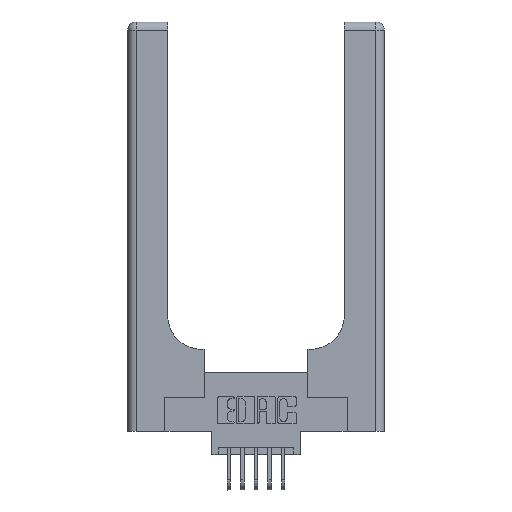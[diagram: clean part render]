
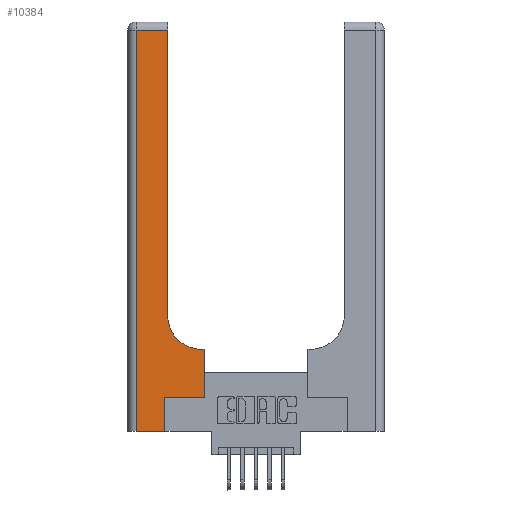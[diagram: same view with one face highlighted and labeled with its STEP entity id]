
A CAD part, top view. The second image highlights one B-rep face of the part: STEP entity #10384.
In plain terms, the highlighted planar face has unit normal (0, 0, 1).
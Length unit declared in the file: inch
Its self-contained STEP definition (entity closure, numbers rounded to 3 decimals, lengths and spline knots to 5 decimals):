
#715 = CARTESIAN_POINT ( 'NONE',  ( 0., 3., 0.37 ) ) ;
#1018 = CARTESIAN_POINT ( 'NONE',  ( 0., 2.94, 0.37 ) ) ;
#1061 = VERTEX_POINT ( 'NONE', #5881 ) ;
#1161 = EDGE_CURVE ( 'NONE', #7354, #1061, #1503, .T. ) ;
#1454 = VERTEX_POINT ( 'NONE', #11573 ) ;
#1472 = VECTOR ( 'NONE', #3896, 39.37008 ) ;
#1502 = CARTESIAN_POINT ( 'NONE',  ( 0.06, 3., 0.37 ) ) ;
#1503 = LINE ( 'NONE', #4188, #1472 ) ;
#1912 = CARTESIAN_POINT ( 'NONE',  ( 0.06, 2.94, 0.37 ) ) ;
#1998 = CARTESIAN_POINT ( 'NONE',  ( 0.269, 0., 0.37 ) ) ;
#2055 = EDGE_CURVE ( 'NONE', #10056, #12913, #4078, .T. ) ;
#2505 = LINE ( 'NONE', #11659, #2764 ) ;
#2760 = CARTESIAN_POINT ( 'NONE',  ( 0.269, 0., 0.37 ) ) ;
#2764 = VECTOR ( 'NONE', #5152, 39.37008 ) ;
#3161 = CARTESIAN_POINT ( 'NONE',  ( 0.5415, 0.85, 0.37 ) ) ;
#3409 = ORIENTED_EDGE ( 'NONE', *, *, #1161, .T. ) ;
#3434 = ORIENTED_EDGE ( 'NONE', *, *, #13379, .T. ) ;
#3467 = DIRECTION ( 'NONE',  ( -1., 0., 0. ) ) ;
#3896 = DIRECTION ( 'NONE',  ( 1., 0., 0. ) ) ;
#3915 = VECTOR ( 'NONE', #4666, 39.37008 ) ;
#4078 = LINE ( 'NONE', #4812, #3915 ) ;
#4188 = CARTESIAN_POINT ( 'NONE',  ( 0.269, 0.25, 0.37 ) ) ;
#4427 = DIRECTION ( 'NONE',  ( 1., 0., 0. ) ) ;
#4574 = ORIENTED_EDGE ( 'NONE', *, *, #10294, .T. ) ;
#4666 = DIRECTION ( 'NONE',  ( 1., 0., 0. ) ) ;
#4812 = CARTESIAN_POINT ( 'NONE',  ( 0., 0., 0.37 ) ) ;
#4821 = ORIENTED_EDGE ( 'NONE', *, *, #6225, .T. ) ;
#5152 = DIRECTION ( 'NONE',  ( -1., 0., 0. ) ) ;
#5512 = LINE ( 'NONE', #5766, #11905 ) ;
#5680 = EDGE_CURVE ( 'NONE', #1061, #14161, #9275, .T. ) ;
#5766 = CARTESIAN_POINT ( 'NONE',  ( 0.2915, 3., 0.37 ) ) ;
#5881 = CARTESIAN_POINT ( 'NONE',  ( 0.5585, 0.25, 0.37 ) ) ;
#6225 = EDGE_CURVE ( 'NONE', #1454, #13155, #10507, .T. ) ;
#6358 = CARTESIAN_POINT ( 'NONE',  ( 0.2915, 0.85, 0.37 ) ) ;
#6363 = VECTOR ( 'NONE', #10239, 39.37008 ) ;
#6426 = CARTESIAN_POINT ( 'NONE',  ( 0.5585, 0.6, 0.37 ) ) ;
#6472 = ORIENTED_EDGE ( 'NONE', *, *, #2055, .T. ) ;
#6473 = LINE ( 'NONE', #1998, #6363 ) ;
#6503 = EDGE_CURVE ( 'NONE', #13155, #10056, #7021, .T. ) ;
#6574 = VECTOR ( 'NONE', #13185, 39.37008 ) ;
#6645 = EDGE_CURVE ( 'NONE', #8983, #9881, #6663, .T. ) ;
#6663 = CIRCLE ( 'NONE', #12162, 0.25 ) ;
#6765 = EDGE_CURVE ( 'NONE', #12913, #7354, #6473, .T. ) ;
#6948 = VECTOR ( 'NONE', #8909, 39.37008 ) ;
#7021 = LINE ( 'NONE', #1502, #6948 ) ;
#7249 = CARTESIAN_POINT ( 'NONE',  ( 0.5585, 0.25, 0.37 ) ) ;
#7354 = VERTEX_POINT ( 'NONE', #10998 ) ;
#8318 = PLANE ( 'NONE',  #12484 ) ;
#8344 = ORIENTED_EDGE ( 'NONE', *, *, #6503, .T. ) ;
#8909 = DIRECTION ( 'NONE',  ( 0., -1., 0. ) ) ;
#8983 = VERTEX_POINT ( 'NONE', #12132 ) ;
#9275 = LINE ( 'NONE', #7249, #6574 ) ;
#9595 = DIRECTION ( 'NONE',  ( -1., 0., 0. ) ) ;
#9866 = ORIENTED_EDGE ( 'NONE', *, *, #6765, .T. ) ;
#9881 = VERTEX_POINT ( 'NONE', #6358 ) ;
#10056 = VERTEX_POINT ( 'NONE', #10915 ) ;
#10239 = DIRECTION ( 'NONE',  ( 0., 1., 0. ) ) ;
#10294 = EDGE_CURVE ( 'NONE', #9881, #1454, #5512, .T. ) ;
#10341 = DIRECTION ( 'NONE',  ( 0., 0., -1. ) ) ;
#10384 = ADVANCED_FACE ( 'NONE', ( #12512 ), #8318, .F. ) ;
#10507 = LINE ( 'NONE', #1018, #10791 ) ;
#10791 = VECTOR ( 'NONE', #9595, 39.37008 ) ;
#10915 = CARTESIAN_POINT ( 'NONE',  ( 0.06, 0., 0.37 ) ) ;
#10998 = CARTESIAN_POINT ( 'NONE',  ( 0.269, 0.25, 0.37 ) ) ;
#11051 = DIRECTION ( 'NONE',  ( 0., 0., -1. ) ) ;
#11573 = CARTESIAN_POINT ( 'NONE',  ( 0.2915, 2.94, 0.37 ) ) ;
#11659 = CARTESIAN_POINT ( 'NONE',  ( 0.2915, 0.6, 0.37 ) ) ;
#11905 = VECTOR ( 'NONE', #12102, 39.37008 ) ;
#12102 = DIRECTION ( 'NONE',  ( 0., 1., 0. ) ) ;
#12132 = CARTESIAN_POINT ( 'NONE',  ( 0.5415, 0.6, 0.37 ) ) ;
#12162 = AXIS2_PLACEMENT_3D ( 'NONE', #3161, #11051, #4427 ) ;
#12484 = AXIS2_PLACEMENT_3D ( 'NONE', #715, #10341, #3467 ) ;
#12512 = FACE_OUTER_BOUND ( 'NONE', #12655, .T. ) ;
#12655 = EDGE_LOOP ( 'NONE', ( #4574, #4821, #8344, #6472, #9866, #3409, #13498, #3434, #14042 ) ) ;
#12913 = VERTEX_POINT ( 'NONE', #2760 ) ;
#13155 = VERTEX_POINT ( 'NONE', #1912 ) ;
#13185 = DIRECTION ( 'NONE',  ( 0., 1., 0. ) ) ;
#13379 = EDGE_CURVE ( 'NONE', #14161, #8983, #2505, .T. ) ;
#13498 = ORIENTED_EDGE ( 'NONE', *, *, #5680, .T. ) ;
#14042 = ORIENTED_EDGE ( 'NONE', *, *, #6645, .T. ) ;
#14161 = VERTEX_POINT ( 'NONE', #6426 ) ;
